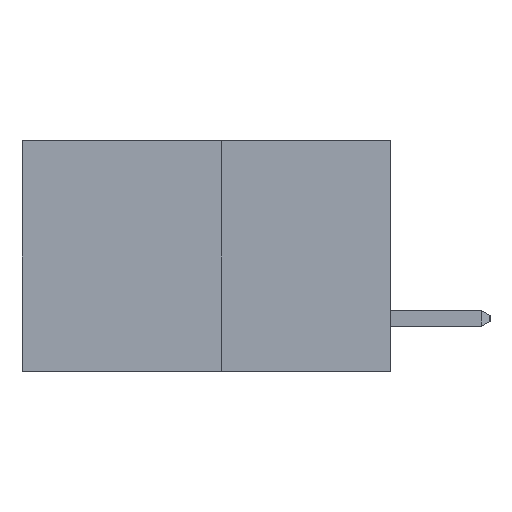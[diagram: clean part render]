
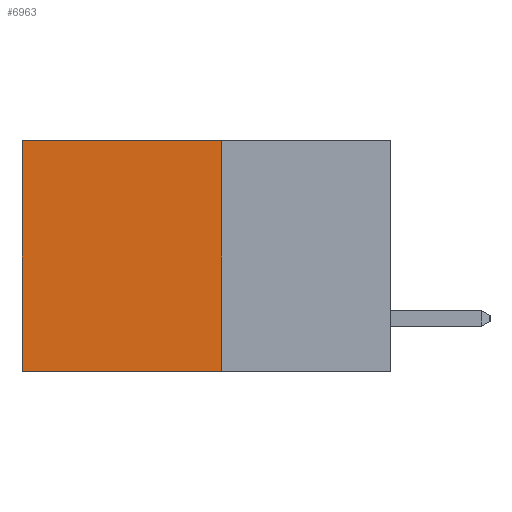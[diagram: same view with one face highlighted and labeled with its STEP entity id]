
A CAD part, left-side view. The second image highlights one B-rep face of the part: STEP entity #6963.
In plain terms, the highlighted planar face has unit normal (-1, 0, 0).
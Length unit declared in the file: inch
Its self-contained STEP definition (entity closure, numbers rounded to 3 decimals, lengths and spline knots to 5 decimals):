
#12 = EDGE_CURVE ( 'NONE', #11826, #9706, #4063, .T. ) ;
#983 = LINE ( 'NONE', #4604, #14890 ) ;
#1115 = ORIENTED_EDGE ( 'NONE', *, *, #12040, .F. ) ;
#2101 = CARTESIAN_POINT ( 'NONE',  ( 0.277, 0.27, -0.37 ) ) ;
#2702 = DIRECTION ( 'NONE',  ( 0., 0., -1. ) ) ;
#3242 = LINE ( 'NONE', #5212, #9779 ) ;
#3527 = CARTESIAN_POINT ( 'NONE',  ( 0.277, 0.27, 0. ) ) ;
#3661 = VECTOR ( 'NONE', #4290, 39.37008 ) ;
#4063 = LINE ( 'NONE', #11869, #3661 ) ;
#4277 = ORIENTED_EDGE ( 'NONE', *, *, #7489, .F. ) ;
#4290 = DIRECTION ( 'NONE',  ( 0., 0., -1. ) ) ;
#4604 = CARTESIAN_POINT ( 'NONE',  ( 0.277, 0.27, -0.37 ) ) ;
#4666 = DIRECTION ( 'NONE',  ( 1., 0., 0. ) ) ;
#5212 = CARTESIAN_POINT ( 'NONE',  ( 0.277, 0.27, 0. ) ) ;
#5771 = FACE_OUTER_BOUND ( 'NONE', #14705, .T. ) ;
#5842 = AXIS2_PLACEMENT_3D ( 'NONE', #11161, #4666, #13752 ) ;
#6598 = VERTEX_POINT ( 'NONE', #2101 ) ;
#6963 = ADVANCED_FACE ( 'NONE', ( #5771 ), #16263, .F. ) ;
#7489 = EDGE_CURVE ( 'NONE', #6598, #9706, #983, .T. ) ;
#7837 = DIRECTION ( 'NONE',  ( 0., 1., 0. ) ) ;
#8030 = VECTOR ( 'NONE', #2702, 39.37008 ) ;
#8512 = DIRECTION ( 'NONE',  ( 0., 1., 0. ) ) ;
#8535 = ORIENTED_EDGE ( 'NONE', *, *, #16316, .T. ) ;
#9706 = VERTEX_POINT ( 'NONE', #14130 ) ;
#9779 = VECTOR ( 'NONE', #7837, 39.37008 ) ;
#11161 = CARTESIAN_POINT ( 'NONE',  ( 0.277, 0.27, -0.37 ) ) ;
#11826 = VERTEX_POINT ( 'NONE', #12778 ) ;
#11850 = CARTESIAN_POINT ( 'NONE',  ( 0.277, 0.27, -0.37 ) ) ;
#11869 = CARTESIAN_POINT ( 'NONE',  ( 0.277, 0.59, -0.37 ) ) ;
#11905 = LINE ( 'NONE', #11850, #8030 ) ;
#12040 = EDGE_CURVE ( 'NONE', #16772, #6598, #11905, .T. ) ;
#12778 = CARTESIAN_POINT ( 'NONE',  ( 0.277, 0.59, 0. ) ) ;
#13752 = DIRECTION ( 'NONE',  ( 0., 0., -1. ) ) ;
#14130 = CARTESIAN_POINT ( 'NONE',  ( 0.277, 0.59, -0.37 ) ) ;
#14232 = ORIENTED_EDGE ( 'NONE', *, *, #12, .T. ) ;
#14705 = EDGE_LOOP ( 'NONE', ( #14232, #4277, #1115, #8535 ) ) ;
#14890 = VECTOR ( 'NONE', #8512, 39.37008 ) ;
#16263 = PLANE ( 'NONE',  #5842 ) ;
#16316 = EDGE_CURVE ( 'NONE', #16772, #11826, #3242, .T. ) ;
#16772 = VERTEX_POINT ( 'NONE', #3527 ) ;
